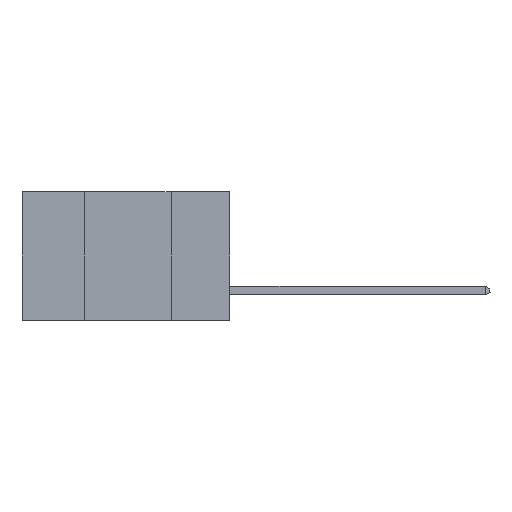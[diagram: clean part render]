
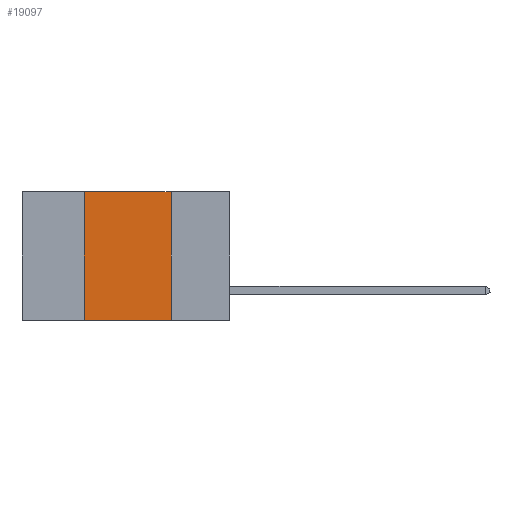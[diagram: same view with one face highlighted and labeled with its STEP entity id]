
A CAD part, left-side view. The second image highlights one B-rep face of the part: STEP entity #19097.
In plain terms, the highlighted planar face has unit normal (-1, 0, 0).
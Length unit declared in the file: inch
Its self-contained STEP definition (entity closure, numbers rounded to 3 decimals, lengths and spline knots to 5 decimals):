
#686 = VERTEX_POINT ( 'NONE', #10829 ) ;
#690 = CARTESIAN_POINT ( 'NONE',  ( 0., 0.42, 0. ) ) ;
#1091 = LINE ( 'NONE', #2609, #22554 ) ;
#1116 = VERTEX_POINT ( 'NONE', #690 ) ;
#1448 = LINE ( 'NONE', #13133, #8359 ) ;
#1627 = DIRECTION ( 'NONE',  ( 0., 0., -1. ) ) ;
#2609 = CARTESIAN_POINT ( 'NONE',  ( 0., 0.6, -0.37 ) ) ;
#4924 = DIRECTION ( 'NONE',  ( 0., -1., 0. ) ) ;
#5263 = EDGE_CURVE ( 'NONE', #686, #1116, #24641, .T. ) ;
#6250 = LINE ( 'NONE', #19617, #10419 ) ;
#6553 = DIRECTION ( 'NONE',  ( 0., -1., 0. ) ) ;
#6582 = VERTEX_POINT ( 'NONE', #23969 ) ;
#8359 = VECTOR ( 'NONE', #6553, 39.37008 ) ;
#9272 = DIRECTION ( 'NONE',  ( 0., 0., -1. ) ) ;
#10419 = VECTOR ( 'NONE', #9272, 39.37008 ) ;
#10829 = CARTESIAN_POINT ( 'NONE',  ( 0., 0.42, -0.37 ) ) ;
#11775 = ORIENTED_EDGE ( 'NONE', *, *, #13647, .F. ) ;
#12977 = CARTESIAN_POINT ( 'NONE',  ( 0., 0.42, 0. ) ) ;
#13133 = CARTESIAN_POINT ( 'NONE',  ( 0., 0.6, 0. ) ) ;
#13647 = EDGE_CURVE ( 'NONE', #6582, #24149, #6250, .T. ) ;
#14639 = ORIENTED_EDGE ( 'NONE', *, *, #19837, .T. ) ;
#14674 = FACE_OUTER_BOUND ( 'NONE', #19913, .T. ) ;
#16952 = ORIENTED_EDGE ( 'NONE', *, *, #5263, .F. ) ;
#17411 = VECTOR ( 'NONE', #26294, 39.37008 ) ;
#17717 = CARTESIAN_POINT ( 'NONE',  ( 0., 0.17, -0.37 ) ) ;
#19097 = ADVANCED_FACE ( 'NONE', ( #14674 ), #26240, .F. ) ;
#19497 = DIRECTION ( 'NONE',  ( 1., 0., 0. ) ) ;
#19617 = CARTESIAN_POINT ( 'NONE',  ( 0., 0.17, 0. ) ) ;
#19837 = EDGE_CURVE ( 'NONE', #686, #24149, #1091, .T. ) ;
#19913 = EDGE_LOOP ( 'NONE', ( #11775, #22775, #16952, #14639 ) ) ;
#20297 = EDGE_CURVE ( 'NONE', #1116, #6582, #1448, .T. ) ;
#22554 = VECTOR ( 'NONE', #4924, 39.37008 ) ;
#22775 = ORIENTED_EDGE ( 'NONE', *, *, #20297, .F. ) ;
#23109 = AXIS2_PLACEMENT_3D ( 'NONE', #28293, #19497, #1627 ) ;
#23969 = CARTESIAN_POINT ( 'NONE',  ( 0., 0.17, 0. ) ) ;
#24149 = VERTEX_POINT ( 'NONE', #17717 ) ;
#24641 = LINE ( 'NONE', #12977, #17411 ) ;
#26240 = PLANE ( 'NONE',  #23109 ) ;
#26294 = DIRECTION ( 'NONE',  ( 0., 0., 1. ) ) ;
#28293 = CARTESIAN_POINT ( 'NONE',  ( 0., 0.6, 0. ) ) ;
